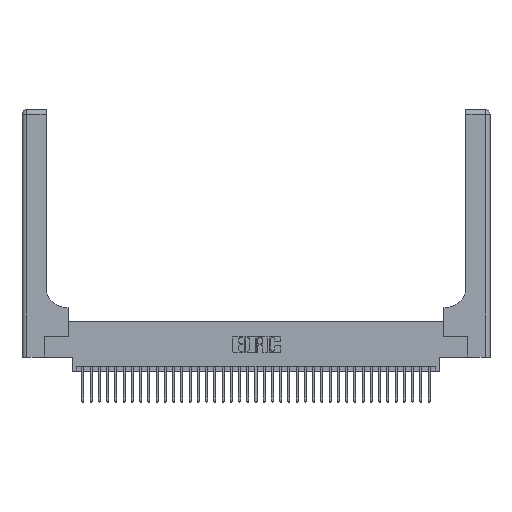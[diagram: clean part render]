
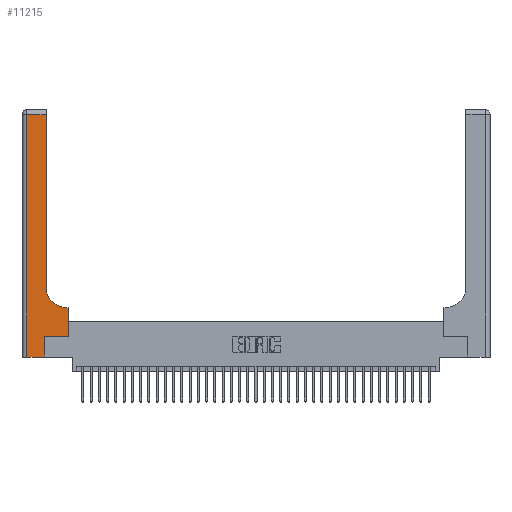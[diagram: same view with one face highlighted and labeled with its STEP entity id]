
A CAD part, top view. The second image highlights one B-rep face of the part: STEP entity #11215.
In plain terms, the highlighted planar face has unit normal (0, 0, 1).
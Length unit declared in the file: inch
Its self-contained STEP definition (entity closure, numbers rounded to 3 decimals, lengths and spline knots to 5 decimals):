
#288 = VECTOR ( 'NONE', #26329, 39.37008 ) ;
#2138 = CARTESIAN_POINT ( 'NONE',  ( 0.06, 3., 0.37 ) ) ;
#2178 = DIRECTION ( 'NONE',  ( 1., 0., 0. ) ) ;
#4221 = LINE ( 'NONE', #35859, #9377 ) ;
#4657 = CARTESIAN_POINT ( 'NONE',  ( 0.06, 2.94, 0.37 ) ) ;
#5018 = DIRECTION ( 'NONE',  ( 0., 1., 0. ) ) ;
#5255 = ORIENTED_EDGE ( 'NONE', *, *, #19868, .T. ) ;
#5437 = EDGE_CURVE ( 'NONE', #12783, #11900, #4221, .T. ) ;
#5459 = LINE ( 'NONE', #17074, #33632 ) ;
#5650 = CARTESIAN_POINT ( 'NONE',  ( 0.5585, 0.6, 0.37 ) ) ;
#6071 = CARTESIAN_POINT ( 'NONE',  ( 0.269, 0., 0.37 ) ) ;
#6883 = EDGE_CURVE ( 'NONE', #36461, #12783, #14404, .T. ) ;
#8019 = CARTESIAN_POINT ( 'NONE',  ( 0., 3., 0.37 ) ) ;
#8302 = CARTESIAN_POINT ( 'NONE',  ( 0.5585, 0.25, 0.37 ) ) ;
#8695 = CARTESIAN_POINT ( 'NONE',  ( 0.5415, 0.85, 0.37 ) ) ;
#8715 = VERTEX_POINT ( 'NONE', #21119 ) ;
#8842 = LINE ( 'NONE', #38432, #288 ) ;
#9060 = EDGE_CURVE ( 'NONE', #27124, #8715, #5459, .T. ) ;
#9216 = CARTESIAN_POINT ( 'NONE',  ( 0.06, 0., 0.37 ) ) ;
#9332 = EDGE_CURVE ( 'NONE', #24555, #31405, #15292, .T. ) ;
#9377 = VECTOR ( 'NONE', #35597, 39.37008 ) ;
#9777 = ORIENTED_EDGE ( 'NONE', *, *, #20001, .T. ) ;
#10886 = DIRECTION ( 'NONE',  ( -1., 0., 0. ) ) ;
#11065 = VECTOR ( 'NONE', #17959, 39.37008 ) ;
#11090 = VECTOR ( 'NONE', #5018, 39.37008 ) ;
#11215 = ADVANCED_FACE ( 'NONE', ( #27600 ), #32884, .F. ) ;
#11900 = VERTEX_POINT ( 'NONE', #36836 ) ;
#12783 = VERTEX_POINT ( 'NONE', #23000 ) ;
#14097 = DIRECTION ( 'NONE',  ( 0., 1., 0. ) ) ;
#14404 = LINE ( 'NONE', #6071, #33231 ) ;
#14448 = DIRECTION ( 'NONE',  ( 0., 0., -1. ) ) ;
#15292 = LINE ( 'NONE', #27774, #16227 ) ;
#15639 = ORIENTED_EDGE ( 'NONE', *, *, #6883, .T. ) ;
#15745 = DIRECTION ( 'NONE',  ( 0., 1., 0. ) ) ;
#16227 = VECTOR ( 'NONE', #14097, 39.37008 ) ;
#17074 = CARTESIAN_POINT ( 'NONE',  ( 0.2915, 0.6, 0.37 ) ) ;
#17959 = DIRECTION ( 'NONE',  ( 0., -1., 0. ) ) ;
#19139 = ORIENTED_EDGE ( 'NONE', *, *, #19414, .T. ) ;
#19414 = EDGE_CURVE ( 'NONE', #31405, #38082, #8842, .T. ) ;
#19868 = EDGE_CURVE ( 'NONE', #11900, #27124, #36510, .T. ) ;
#20001 = EDGE_CURVE ( 'NONE', #8715, #24555, #35515, .T. ) ;
#20218 = CARTESIAN_POINT ( 'NONE',  ( 0.2915, 2.94, 0.37 ) ) ;
#21119 = CARTESIAN_POINT ( 'NONE',  ( 0.5415, 0.6, 0.37 ) ) ;
#21229 = EDGE_CURVE ( 'NONE', #38082, #32876, #34540, .T. ) ;
#22056 = AXIS2_PLACEMENT_3D ( 'NONE', #8019, #25739, #10886 ) ;
#23000 = CARTESIAN_POINT ( 'NONE',  ( 0.269, 0.25, 0.37 ) ) ;
#24088 = ORIENTED_EDGE ( 'NONE', *, *, #9332, .T. ) ;
#24555 = VERTEX_POINT ( 'NONE', #36443 ) ;
#25233 = ORIENTED_EDGE ( 'NONE', *, *, #9060, .T. ) ;
#25739 = DIRECTION ( 'NONE',  ( 0., 0., -1. ) ) ;
#26329 = DIRECTION ( 'NONE',  ( -1., 0., 0. ) ) ;
#27124 = VERTEX_POINT ( 'NONE', #5650 ) ;
#27600 = FACE_OUTER_BOUND ( 'NONE', #37122, .T. ) ;
#27774 = CARTESIAN_POINT ( 'NONE',  ( 0.2915, 3., 0.37 ) ) ;
#28863 = CARTESIAN_POINT ( 'NONE',  ( 0.269, 0., 0.37 ) ) ;
#29127 = DIRECTION ( 'NONE',  ( -1., 0., 0. ) ) ;
#30459 = DIRECTION ( 'NONE',  ( 1., 0., 0. ) ) ;
#30585 = AXIS2_PLACEMENT_3D ( 'NONE', #8695, #14448, #30459 ) ;
#31405 = VERTEX_POINT ( 'NONE', #20218 ) ;
#31531 = VECTOR ( 'NONE', #2178, 39.37008 ) ;
#32742 = ORIENTED_EDGE ( 'NONE', *, *, #33382, .T. ) ;
#32876 = VERTEX_POINT ( 'NONE', #9216 ) ;
#32884 = PLANE ( 'NONE',  #22056 ) ;
#33011 = ORIENTED_EDGE ( 'NONE', *, *, #21229, .T. ) ;
#33231 = VECTOR ( 'NONE', #15745, 39.37008 ) ;
#33382 = EDGE_CURVE ( 'NONE', #32876, #36461, #36278, .T. ) ;
#33632 = VECTOR ( 'NONE', #29127, 39.37008 ) ;
#34091 = ORIENTED_EDGE ( 'NONE', *, *, #5437, .T. ) ;
#34540 = LINE ( 'NONE', #2138, #11065 ) ;
#35515 = CIRCLE ( 'NONE', #30585, 0.25 ) ;
#35559 = CARTESIAN_POINT ( 'NONE',  ( 0., 0., 0.37 ) ) ;
#35597 = DIRECTION ( 'NONE',  ( 1., 0., 0. ) ) ;
#35859 = CARTESIAN_POINT ( 'NONE',  ( 0.269, 0.25, 0.37 ) ) ;
#36278 = LINE ( 'NONE', #35559, #31531 ) ;
#36443 = CARTESIAN_POINT ( 'NONE',  ( 0.2915, 0.85, 0.37 ) ) ;
#36461 = VERTEX_POINT ( 'NONE', #28863 ) ;
#36510 = LINE ( 'NONE', #8302, #11090 ) ;
#36836 = CARTESIAN_POINT ( 'NONE',  ( 0.5585, 0.25, 0.37 ) ) ;
#37122 = EDGE_LOOP ( 'NONE', ( #24088, #19139, #33011, #32742, #15639, #34091, #5255, #25233, #9777 ) ) ;
#38082 = VERTEX_POINT ( 'NONE', #4657 ) ;
#38432 = CARTESIAN_POINT ( 'NONE',  ( 0., 2.94, 0.37 ) ) ;
